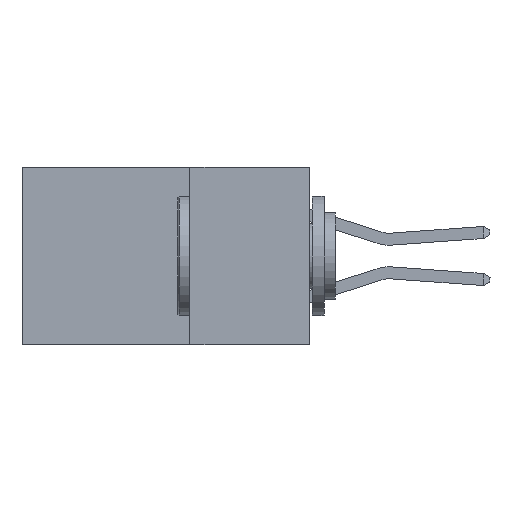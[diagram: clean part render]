
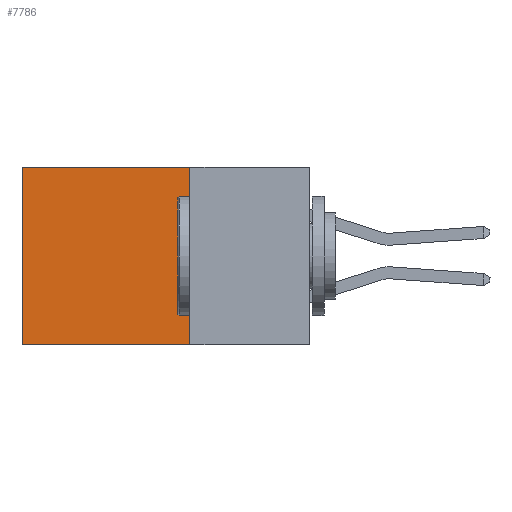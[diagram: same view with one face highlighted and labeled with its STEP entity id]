
A CAD part, left-side view. The second image highlights one B-rep face of the part: STEP entity #7786.
In plain terms, the highlighted planar face has unit normal (-1, 0, 0).
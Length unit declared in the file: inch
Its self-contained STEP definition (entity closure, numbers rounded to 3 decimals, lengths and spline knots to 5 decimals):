
#576 = EDGE_CURVE ( 'NONE', #10518, #15207, #7994, .T. ) ;
#1824 = DIRECTION ( 'NONE',  ( 0., 1., 0. ) ) ;
#1994 = CARTESIAN_POINT ( 'NONE',  ( 0.2615, 0.25, 0. ) ) ;
#3183 = LINE ( 'NONE', #1994, #21951 ) ;
#3542 = VERTEX_POINT ( 'NONE', #17133 ) ;
#4029 = DIRECTION ( 'NONE',  ( 0., 0., -1. ) ) ;
#4210 = DIRECTION ( 'NONE',  ( 1., 0., 0. ) ) ;
#4636 = EDGE_LOOP ( 'NONE', ( #13267, #10821, #15320, #17236 ) ) ;
#4746 = PLANE ( 'NONE',  #20283 ) ;
#5767 = CARTESIAN_POINT ( 'NONE',  ( 0.2615, 0.25, -0.37 ) ) ;
#6603 = CARTESIAN_POINT ( 'NONE',  ( 0.2615, 0.6, 0. ) ) ;
#7786 = ADVANCED_FACE ( 'NONE', ( #15701 ), #4746, .F. ) ;
#7994 = LINE ( 'NONE', #16028, #12901 ) ;
#8034 = DIRECTION ( 'NONE',  ( 0., 1., 0. ) ) ;
#8995 = EDGE_CURVE ( 'NONE', #3542, #10518, #13687, .T. ) ;
#10477 = CARTESIAN_POINT ( 'NONE',  ( 0.2615, 0.6, -0.37 ) ) ;
#10518 = VERTEX_POINT ( 'NONE', #11856 ) ;
#10821 = ORIENTED_EDGE ( 'NONE', *, *, #576, .F. ) ;
#11298 = EDGE_CURVE ( 'NONE', #3542, #13525, #3183, .T. ) ;
#11856 = CARTESIAN_POINT ( 'NONE',  ( 0.2615, 0.25, -0.37 ) ) ;
#12320 = DIRECTION ( 'NONE',  ( 0., 0., -1. ) ) ;
#12558 = CARTESIAN_POINT ( 'NONE',  ( 0.2615, 0.6, -0.37 ) ) ;
#12898 = EDGE_CURVE ( 'NONE', #13525, #15207, #22701, .T. ) ;
#12901 = VECTOR ( 'NONE', #8034, 39.37008 ) ;
#13267 = ORIENTED_EDGE ( 'NONE', *, *, #12898, .T. ) ;
#13525 = VERTEX_POINT ( 'NONE', #6603 ) ;
#13687 = LINE ( 'NONE', #18198, #17877 ) ;
#13763 = VECTOR ( 'NONE', #12320, 39.37008 ) ;
#15207 = VERTEX_POINT ( 'NONE', #12558 ) ;
#15320 = ORIENTED_EDGE ( 'NONE', *, *, #8995, .F. ) ;
#15701 = FACE_OUTER_BOUND ( 'NONE', #4636, .T. ) ;
#16028 = CARTESIAN_POINT ( 'NONE',  ( 0.2615, 0.25, -0.37 ) ) ;
#17133 = CARTESIAN_POINT ( 'NONE',  ( 0.2615, 0.25, 0. ) ) ;
#17236 = ORIENTED_EDGE ( 'NONE', *, *, #11298, .T. ) ;
#17495 = DIRECTION ( 'NONE',  ( 0., 0., -1. ) ) ;
#17877 = VECTOR ( 'NONE', #17495, 39.37008 ) ;
#18198 = CARTESIAN_POINT ( 'NONE',  ( 0.2615, 0.25, -0.37 ) ) ;
#20283 = AXIS2_PLACEMENT_3D ( 'NONE', #5767, #4210, #4029 ) ;
#21951 = VECTOR ( 'NONE', #1824, 39.37008 ) ;
#22701 = LINE ( 'NONE', #10477, #13763 ) ;
